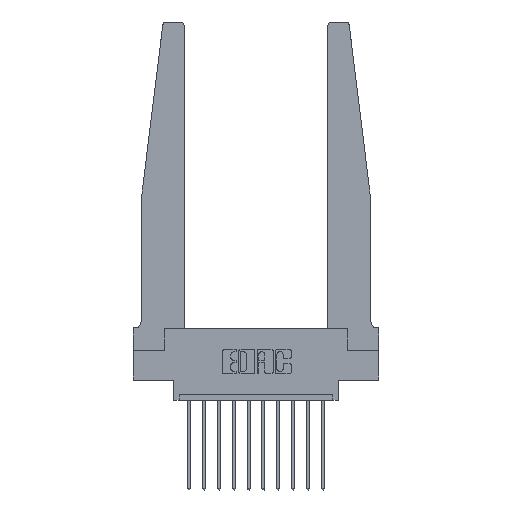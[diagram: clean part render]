
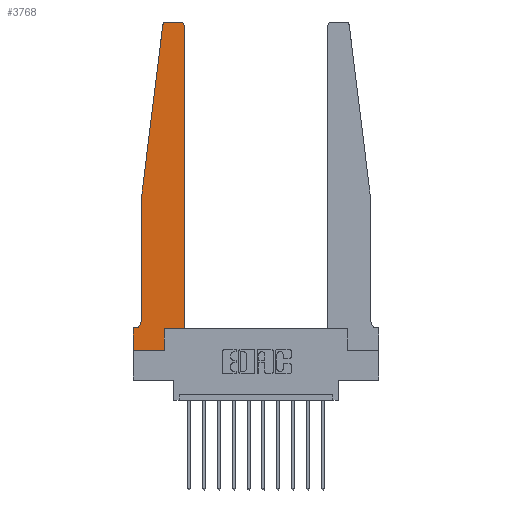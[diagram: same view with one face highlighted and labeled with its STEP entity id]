
A CAD part, top view. The second image highlights one B-rep face of the part: STEP entity #3768.
In plain terms, the highlighted planar face has unit normal (0, 0, 1).
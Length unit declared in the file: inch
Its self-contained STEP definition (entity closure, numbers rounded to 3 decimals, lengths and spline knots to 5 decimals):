
#385 = EDGE_CURVE ( 'NONE', #2357, #11290, #9641, .T. ) ;
#600 = VECTOR ( 'NONE', #2851, 39.37008 ) ;
#608 = PLANE ( 'NONE',  #5637 ) ;
#622 = EDGE_CURVE ( 'NONE', #6438, #10337, #7724, .T. ) ;
#651 = CARTESIAN_POINT ( 'NONE',  ( 0.2605, 0.18, 0.37 ) ) ;
#1087 = CARTESIAN_POINT ( 'NONE',  ( 0.395, 2.72, 0.37 ) ) ;
#1142 = CARTESIAN_POINT ( 'NONE',  ( 0., 0.1875, 0.37 ) ) ;
#1297 = VERTEX_POINT ( 'NONE', #7750 ) ;
#1350 = LINE ( 'NONE', #11148, #15378 ) ;
#1552 = CARTESIAN_POINT ( 'NONE',  ( 0.2605, 0., 0.37 ) ) ;
#1594 = ORIENTED_EDGE ( 'NONE', *, *, #8028, .T. ) ;
#1612 = DIRECTION ( 'NONE',  ( 0., 1., 0. ) ) ;
#1779 = VECTOR ( 'NONE', #7373, 39.37008 ) ;
#1856 = EDGE_CURVE ( 'NONE', #3572, #14567, #11594, .T. ) ;
#2232 = CARTESIAN_POINT ( 'NONE',  ( 0.25, 2.75, 0.37 ) ) ;
#2244 = CARTESIAN_POINT ( 'NONE',  ( 0.065, 1.25, 0.37 ) ) ;
#2347 = VERTEX_POINT ( 'NONE', #7313 ) ;
#2357 = VERTEX_POINT ( 'NONE', #1142 ) ;
#2697 = EDGE_CURVE ( 'NONE', #12362, #8255, #7296, .T. ) ;
#2851 = DIRECTION ( 'NONE',  ( 0., 1., 0. ) ) ;
#2968 = DIRECTION ( 'NONE',  ( -0.122, -0.992, 0. ) ) ;
#2993 = DIRECTION ( 'NONE',  ( 1., 0., 0. ) ) ;
#3061 = VECTOR ( 'NONE', #1612, 39.37008 ) ;
#3082 = CARTESIAN_POINT ( 'NONE',  ( 0.425, 0.18, 0.37 ) ) ;
#3126 = CARTESIAN_POINT ( 'NONE',  ( 0.27653, 2.72, 0.37 ) ) ;
#3274 = LINE ( 'NONE', #2232, #5945 ) ;
#3312 = AXIS2_PLACEMENT_3D ( 'NONE', #1087, #15742, #13274 ) ;
#3481 = EDGE_CURVE ( 'NONE', #3746, #2347, #12815, .T. ) ;
#3572 = VERTEX_POINT ( 'NONE', #15590 ) ;
#3746 = VERTEX_POINT ( 'NONE', #6770 ) ;
#3768 = ADVANCED_FACE ( 'NONE', ( #4360 ), #608, .T. ) ;
#4084 = LINE ( 'NONE', #8997, #14108 ) ;
#4128 = AXIS2_PLACEMENT_3D ( 'NONE', #3126, #8041, #11886 ) ;
#4360 = FACE_OUTER_BOUND ( 'NONE', #11555, .T. ) ;
#4800 = CARTESIAN_POINT ( 'NONE',  ( 0.065, 0.2375, 0.37 ) ) ;
#4932 = EDGE_CURVE ( 'NONE', #1297, #3746, #6851, .T. ) ;
#5038 = VECTOR ( 'NONE', #2968, 39.37008 ) ;
#5411 = LINE ( 'NONE', #14959, #10451 ) ;
#5637 = AXIS2_PLACEMENT_3D ( 'NONE', #6531, #12724, #2993 ) ;
#5880 = ORIENTED_EDGE ( 'NONE', *, *, #9303, .T. ) ;
#5945 = VECTOR ( 'NONE', #8196, 39.37008 ) ;
#5964 = EDGE_CURVE ( 'NONE', #11290, #6438, #5411, .T. ) ;
#6086 = ORIENTED_EDGE ( 'NONE', *, *, #1856, .T. ) ;
#6194 = ORIENTED_EDGE ( 'NONE', *, *, #4932, .T. ) ;
#6438 = VERTEX_POINT ( 'NONE', #1552 ) ;
#6531 = CARTESIAN_POINT ( 'NONE',  ( 0., 0.1875, 0.37 ) ) ;
#6555 = DIRECTION ( 'NONE',  ( 0., 0., -1. ) ) ;
#6770 = CARTESIAN_POINT ( 'NONE',  ( 0.425, 2.72, 0.37 ) ) ;
#6851 = LINE ( 'NONE', #3082, #600 ) ;
#7234 = CARTESIAN_POINT ( 'NONE',  ( 0.015, 0.1875, 0.37 ) ) ;
#7296 = LINE ( 'NONE', #13230, #1779 ) ;
#7313 = CARTESIAN_POINT ( 'NONE',  ( 0.395, 2.75, 0.37 ) ) ;
#7354 = DIRECTION ( 'NONE',  ( 1., 0., 0. ) ) ;
#7373 = DIRECTION ( 'NONE',  ( 0., -1., 0. ) ) ;
#7581 = ORIENTED_EDGE ( 'NONE', *, *, #5964, .T. ) ;
#7724 = LINE ( 'NONE', #12771, #3061 ) ;
#7750 = CARTESIAN_POINT ( 'NONE',  ( 0.425, 0.18, 0.37 ) ) ;
#8019 = ORIENTED_EDGE ( 'NONE', *, *, #12818, .T. ) ;
#8028 = EDGE_CURVE ( 'NONE', #14567, #12362, #15087, .T. ) ;
#8036 = DIRECTION ( 'NONE',  ( -1., 0., 0. ) ) ;
#8041 = DIRECTION ( 'NONE',  ( 0., 0., 1. ) ) ;
#8196 = DIRECTION ( 'NONE',  ( -1., 0., 0. ) ) ;
#8255 = VERTEX_POINT ( 'NONE', #4800 ) ;
#8659 = ORIENTED_EDGE ( 'NONE', *, *, #15157, .T. ) ;
#8997 = CARTESIAN_POINT ( 'NONE',  ( 0.065, 0.1875, 0.37 ) ) ;
#9016 = ORIENTED_EDGE ( 'NONE', *, *, #385, .T. ) ;
#9062 = DIRECTION ( 'NONE',  ( 1., 0., 0. ) ) ;
#9292 = CARTESIAN_POINT ( 'NONE',  ( 0.015, 0.2375, 0.37 ) ) ;
#9303 = EDGE_CURVE ( 'NONE', #2347, #3572, #3274, .T. ) ;
#9398 = ORIENTED_EDGE ( 'NONE', *, *, #622, .T. ) ;
#9454 = CIRCLE ( 'NONE', #10755, 0.05 ) ;
#9641 = LINE ( 'NONE', #11163, #11386 ) ;
#10337 = VERTEX_POINT ( 'NONE', #651 ) ;
#10451 = VECTOR ( 'NONE', #7354, 39.37008 ) ;
#10755 = AXIS2_PLACEMENT_3D ( 'NONE', #9292, #6555, #11643 ) ;
#11148 = CARTESIAN_POINT ( 'NONE',  ( 0.425, 0.18, 0.37 ) ) ;
#11163 = CARTESIAN_POINT ( 'NONE',  ( 0., 0., 0.37 ) ) ;
#11259 = ORIENTED_EDGE ( 'NONE', *, *, #14792, .T. ) ;
#11290 = VERTEX_POINT ( 'NONE', #12991 ) ;
#11386 = VECTOR ( 'NONE', #12366, 39.37008 ) ;
#11555 = EDGE_LOOP ( 'NONE', ( #5880, #6086, #1594, #15216, #8019, #11259, #9016, #7581, #9398, #8659, #6194, #12122 ) ) ;
#11594 = CIRCLE ( 'NONE', #4128, 0.03 ) ;
#11643 = DIRECTION ( 'NONE',  ( -1., 0., 0. ) ) ;
#11886 = DIRECTION ( 'NONE',  ( 1., 0., 0. ) ) ;
#12122 = ORIENTED_EDGE ( 'NONE', *, *, #3481, .T. ) ;
#12362 = VERTEX_POINT ( 'NONE', #2244 ) ;
#12366 = DIRECTION ( 'NONE',  ( 0., -1., 0. ) ) ;
#12724 = DIRECTION ( 'NONE',  ( 0., 0., 1. ) ) ;
#12771 = CARTESIAN_POINT ( 'NONE',  ( 0.2605, 0.18, 0.37 ) ) ;
#12815 = CIRCLE ( 'NONE', #3312, 0.03 ) ;
#12818 = EDGE_CURVE ( 'NONE', #8255, #13374, #9454, .T. ) ;
#12991 = CARTESIAN_POINT ( 'NONE',  ( 0., 0., 0.37 ) ) ;
#13230 = CARTESIAN_POINT ( 'NONE',  ( 0.065, 1.25, 0.37 ) ) ;
#13274 = DIRECTION ( 'NONE',  ( 1., 0., 0. ) ) ;
#13374 = VERTEX_POINT ( 'NONE', #7234 ) ;
#13406 = CARTESIAN_POINT ( 'NONE',  ( 0.24675, 2.72367, 0.37 ) ) ;
#13812 = CARTESIAN_POINT ( 'NONE',  ( 0.065, 1.25, 0.37 ) ) ;
#14108 = VECTOR ( 'NONE', #8036, 39.37008 ) ;
#14567 = VERTEX_POINT ( 'NONE', #13406 ) ;
#14792 = EDGE_CURVE ( 'NONE', #13374, #2357, #4084, .T. ) ;
#14959 = CARTESIAN_POINT ( 'NONE',  ( 0., 0., 0.37 ) ) ;
#15087 = LINE ( 'NONE', #13812, #5038 ) ;
#15157 = EDGE_CURVE ( 'NONE', #10337, #1297, #1350, .T. ) ;
#15216 = ORIENTED_EDGE ( 'NONE', *, *, #2697, .T. ) ;
#15378 = VECTOR ( 'NONE', #9062, 39.37008 ) ;
#15590 = CARTESIAN_POINT ( 'NONE',  ( 0.27653, 2.75, 0.37 ) ) ;
#15742 = DIRECTION ( 'NONE',  ( 0., 0., 1. ) ) ;
